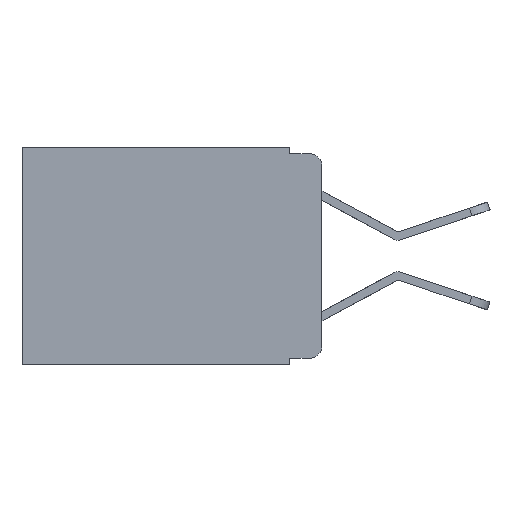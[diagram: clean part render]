
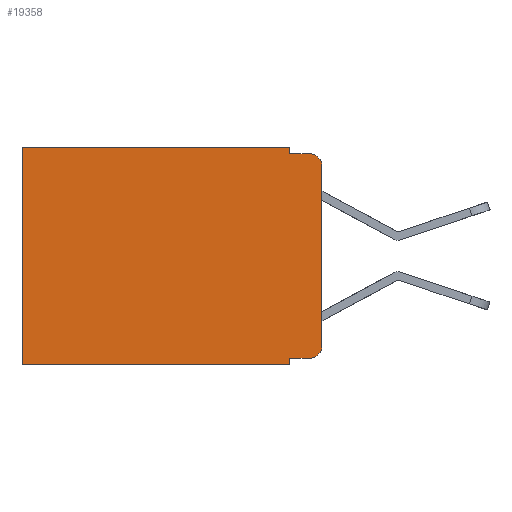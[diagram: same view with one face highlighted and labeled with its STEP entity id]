
A CAD part, left-side view. The second image highlights one B-rep face of the part: STEP entity #19358.
In plain terms, the highlighted planar face has unit normal (-1, 0, 0).
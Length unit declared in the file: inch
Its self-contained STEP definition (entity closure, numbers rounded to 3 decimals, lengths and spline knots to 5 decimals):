
#237 = VERTEX_POINT ( 'NONE', #13044 ) ;
#394 = DIRECTION ( 'NONE',  ( 0., 0., -1. ) ) ;
#500 = VECTOR ( 'NONE', #19558, 39.37008 ) ;
#885 = ORIENTED_EDGE ( 'NONE', *, *, #15789, .T. ) ;
#907 = VECTOR ( 'NONE', #15413, 39.37008 ) ;
#970 = FACE_OUTER_BOUND ( 'NONE', #4651, .T. ) ;
#1333 = CARTESIAN_POINT ( 'NONE',  ( 0.298, 0., -0.03 ) ) ;
#2690 = PLANE ( 'NONE',  #14414 ) ;
#2892 = CARTESIAN_POINT ( 'NONE',  ( 0.298, 0.02, -0.333 ) ) ;
#2988 = DIRECTION ( 'NONE',  ( 0., 0., -1. ) ) ;
#3208 = LINE ( 'NONE', #17370, #19734 ) ;
#3226 = VERTEX_POINT ( 'NONE', #18004 ) ;
#3754 = AXIS2_PLACEMENT_3D ( 'NONE', #5692, #16847, #7306 ) ;
#4380 = CARTESIAN_POINT ( 'NONE',  ( 0.298, 0.051, -0.01 ) ) ;
#4522 = CARTESIAN_POINT ( 'NONE',  ( 0.298, 0.051, -0.343 ) ) ;
#4590 = CARTESIAN_POINT ( 'NONE',  ( 0.298, 0., 0. ) ) ;
#4651 = EDGE_LOOP ( 'NONE', ( #20369, #9205, #9476, #16644, #885, #15668, #20387, #19175, #7180, #9720 ) ) ;
#5190 = EDGE_CURVE ( 'NONE', #16498, #237, #19406, .T. ) ;
#5692 = CARTESIAN_POINT ( 'NONE',  ( 0.298, 0.02, -0.03 ) ) ;
#5985 = LINE ( 'NONE', #20215, #907 ) ;
#6294 = EDGE_CURVE ( 'NONE', #18718, #16498, #17375, .T. ) ;
#6435 = LINE ( 'NONE', #4590, #11208 ) ;
#6564 = CARTESIAN_POINT ( 'NONE',  ( 0.298, 0.051, -0.01 ) ) ;
#7168 = CARTESIAN_POINT ( 'NONE',  ( 0.298, 0.051, 0. ) ) ;
#7180 = ORIENTED_EDGE ( 'NONE', *, *, #6294, .T. ) ;
#7194 = CARTESIAN_POINT ( 'NONE',  ( 0.298, 0.02, -0.313 ) ) ;
#7306 = DIRECTION ( 'NONE',  ( 0., 0., -1. ) ) ;
#7361 = EDGE_CURVE ( 'NONE', #18718, #15836, #3208, .T. ) ;
#7854 = VERTEX_POINT ( 'NONE', #10607 ) ;
#8176 = DIRECTION ( 'NONE',  ( 0., -1., 0. ) ) ;
#8437 = EDGE_CURVE ( 'NONE', #7854, #19810, #5985, .T. ) ;
#8695 = VECTOR ( 'NONE', #394, 39.37008 ) ;
#8808 = DIRECTION ( 'NONE',  ( 0., 0., -1. ) ) ;
#9030 = VERTEX_POINT ( 'NONE', #4380 ) ;
#9205 = ORIENTED_EDGE ( 'NONE', *, *, #13760, .T. ) ;
#9223 = CARTESIAN_POINT ( 'NONE',  ( 0.298, 0., 0. ) ) ;
#9476 = ORIENTED_EDGE ( 'NONE', *, *, #10585, .F. ) ;
#9525 = EDGE_CURVE ( 'NONE', #17885, #9030, #12926, .T. ) ;
#9720 = ORIENTED_EDGE ( 'NONE', *, *, #5190, .T. ) ;
#10250 = CARTESIAN_POINT ( 'NONE',  ( 0.298, 0., -0.343 ) ) ;
#10380 = VECTOR ( 'NONE', #13563, 39.37008 ) ;
#10585 = EDGE_CURVE ( 'NONE', #9030, #3226, #10922, .T. ) ;
#10607 = CARTESIAN_POINT ( 'NONE',  ( 0.298, 0.473, 0. ) ) ;
#10829 = DIRECTION ( 'NONE',  ( 0., 0., -1. ) ) ;
#10922 = LINE ( 'NONE', #6564, #18862 ) ;
#11208 = VECTOR ( 'NONE', #17369, 39.37008 ) ;
#11694 = VECTOR ( 'NONE', #18758, 39.37008 ) ;
#12082 = AXIS2_PLACEMENT_3D ( 'NONE', #7194, #18327, #8808 ) ;
#12444 = CARTESIAN_POINT ( 'NONE',  ( 0.298, 0.051, -0.333 ) ) ;
#12680 = LINE ( 'NONE', #18688, #11694 ) ;
#12926 = LINE ( 'NONE', #7168, #8695 ) ;
#13044 = CARTESIAN_POINT ( 'NONE',  ( 0.298, 0., -0.313 ) ) ;
#13563 = DIRECTION ( 'NONE',  ( 0., 1., 0. ) ) ;
#13760 = EDGE_CURVE ( 'NONE', #17210, #3226, #19201, .T. ) ;
#14414 = AXIS2_PLACEMENT_3D ( 'NONE', #9223, #20323, #10829 ) ;
#14529 = CARTESIAN_POINT ( 'NONE',  ( 0.298, 0.051, 0. ) ) ;
#15078 = LINE ( 'NONE', #10250, #10380 ) ;
#15413 = DIRECTION ( 'NONE',  ( 0., 0., -1. ) ) ;
#15668 = ORIENTED_EDGE ( 'NONE', *, *, #8437, .T. ) ;
#15789 = EDGE_CURVE ( 'NONE', #17885, #7854, #12680, .T. ) ;
#15836 = VERTEX_POINT ( 'NONE', #4522 ) ;
#15885 = EDGE_CURVE ( 'NONE', #17210, #237, #6435, .T. ) ;
#15958 = CARTESIAN_POINT ( 'NONE',  ( 0.298, 0.473, -0.343 ) ) ;
#16341 = CARTESIAN_POINT ( 'NONE',  ( 0.298, 0.051, -0.333 ) ) ;
#16498 = VERTEX_POINT ( 'NONE', #2892 ) ;
#16644 = ORIENTED_EDGE ( 'NONE', *, *, #9525, .F. ) ;
#16847 = DIRECTION ( 'NONE',  ( -1., 0., 0. ) ) ;
#17210 = VERTEX_POINT ( 'NONE', #1333 ) ;
#17369 = DIRECTION ( 'NONE',  ( 0., 0., -1. ) ) ;
#17370 = CARTESIAN_POINT ( 'NONE',  ( 0.298, 0.051, 0. ) ) ;
#17375 = LINE ( 'NONE', #16341, #500 ) ;
#17885 = VERTEX_POINT ( 'NONE', #14529 ) ;
#18004 = CARTESIAN_POINT ( 'NONE',  ( 0.298, 0.02, -0.01 ) ) ;
#18327 = DIRECTION ( 'NONE',  ( -1., 0., 0. ) ) ;
#18688 = CARTESIAN_POINT ( 'NONE',  ( 0.298, 0., 0. ) ) ;
#18718 = VERTEX_POINT ( 'NONE', #12444 ) ;
#18758 = DIRECTION ( 'NONE',  ( 0., 1., 0. ) ) ;
#18862 = VECTOR ( 'NONE', #8176, 39.37008 ) ;
#19175 = ORIENTED_EDGE ( 'NONE', *, *, #7361, .F. ) ;
#19201 = CIRCLE ( 'NONE', #3754, 0.02 ) ;
#19358 = ADVANCED_FACE ( 'NONE', ( #970 ), #2690, .F. ) ;
#19406 = CIRCLE ( 'NONE', #12082, 0.02 ) ;
#19558 = DIRECTION ( 'NONE',  ( 0., -1., 0. ) ) ;
#19734 = VECTOR ( 'NONE', #2988, 39.37008 ) ;
#19810 = VERTEX_POINT ( 'NONE', #15958 ) ;
#20215 = CARTESIAN_POINT ( 'NONE',  ( 0.298, 0.473, 0. ) ) ;
#20323 = DIRECTION ( 'NONE',  ( 1., 0., 0. ) ) ;
#20369 = ORIENTED_EDGE ( 'NONE', *, *, #15885, .F. ) ;
#20387 = ORIENTED_EDGE ( 'NONE', *, *, #20798, .F. ) ;
#20798 = EDGE_CURVE ( 'NONE', #15836, #19810, #15078, .T. ) ;
